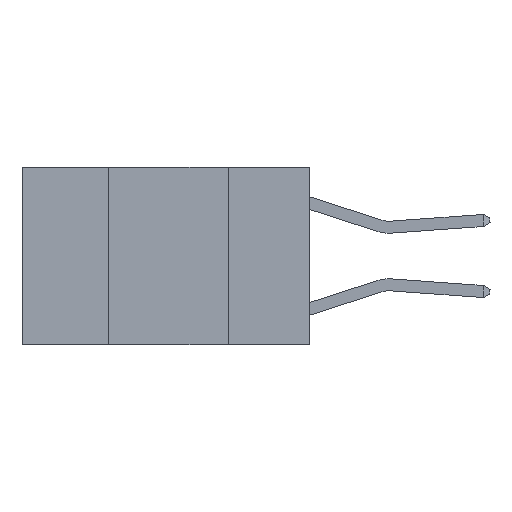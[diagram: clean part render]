
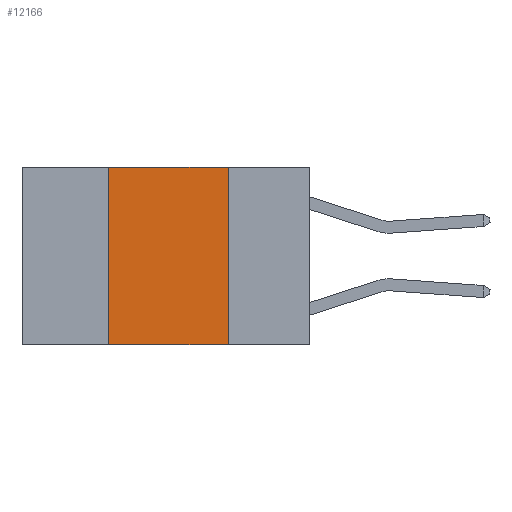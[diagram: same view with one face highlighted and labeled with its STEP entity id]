
A CAD part, left-side view. The second image highlights one B-rep face of the part: STEP entity #12166.
In plain terms, the highlighted planar face has unit normal (-1, 0, 0).
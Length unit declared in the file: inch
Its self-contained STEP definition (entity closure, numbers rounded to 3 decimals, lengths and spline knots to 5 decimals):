
#46 = EDGE_LOOP ( 'NONE', ( #12230, #6119, #9748, #11374 ) ) ;
#489 = EDGE_CURVE ( 'NONE', #6655, #13834, #14466, .T. ) ;
#529 = EDGE_CURVE ( 'NONE', #4726, #6655, #6448, .T. ) ;
#545 = CARTESIAN_POINT ( 'NONE',  ( 0., 0.17, -0.37 ) ) ;
#640 = EDGE_CURVE ( 'NONE', #3314, #13834, #3824, .T. ) ;
#868 = DIRECTION ( 'NONE',  ( 0., 0., -1. ) ) ;
#955 = AXIS2_PLACEMENT_3D ( 'NONE', #13529, #3390, #14388 ) ;
#1019 = CARTESIAN_POINT ( 'NONE',  ( 0., 0.17, 0. ) ) ;
#1156 = PLANE ( 'NONE',  #955 ) ;
#1619 = CARTESIAN_POINT ( 'NONE',  ( 0., 0.17, 0. ) ) ;
#2082 = VECTOR ( 'NONE', #2790, 39.37008 ) ;
#2553 = VECTOR ( 'NONE', #868, 39.37008 ) ;
#2790 = DIRECTION ( 'NONE',  ( 0., -1., 0. ) ) ;
#2953 = CARTESIAN_POINT ( 'NONE',  ( 0., 0.6, 0. ) ) ;
#3314 = VERTEX_POINT ( 'NONE', #9602 ) ;
#3390 = DIRECTION ( 'NONE',  ( 1., 0., 0. ) ) ;
#3824 = LINE ( 'NONE', #13140, #2082 ) ;
#4726 = VERTEX_POINT ( 'NONE', #8680 ) ;
#6119 = ORIENTED_EDGE ( 'NONE', *, *, #529, .F. ) ;
#6448 = LINE ( 'NONE', #2953, #12219 ) ;
#6655 = VERTEX_POINT ( 'NONE', #1619 ) ;
#6734 = LINE ( 'NONE', #14311, #14446 ) ;
#7844 = FACE_OUTER_BOUND ( 'NONE', #46, .T. ) ;
#8495 = EDGE_CURVE ( 'NONE', #3314, #4726, #6734, .T. ) ;
#8680 = CARTESIAN_POINT ( 'NONE',  ( 0., 0.42, 0. ) ) ;
#9602 = CARTESIAN_POINT ( 'NONE',  ( 0., 0.42, -0.37 ) ) ;
#9748 = ORIENTED_EDGE ( 'NONE', *, *, #8495, .F. ) ;
#9950 = DIRECTION ( 'NONE',  ( 0., 0., 1. ) ) ;
#11374 = ORIENTED_EDGE ( 'NONE', *, *, #640, .T. ) ;
#12166 = ADVANCED_FACE ( 'NONE', ( #7844 ), #1156, .F. ) ;
#12219 = VECTOR ( 'NONE', #14033, 39.37008 ) ;
#12230 = ORIENTED_EDGE ( 'NONE', *, *, #489, .F. ) ;
#13140 = CARTESIAN_POINT ( 'NONE',  ( 0., 0.6, -0.37 ) ) ;
#13529 = CARTESIAN_POINT ( 'NONE',  ( 0., 0.6, 0. ) ) ;
#13834 = VERTEX_POINT ( 'NONE', #545 ) ;
#14033 = DIRECTION ( 'NONE',  ( 0., -1., 0. ) ) ;
#14311 = CARTESIAN_POINT ( 'NONE',  ( 0., 0.42, 0. ) ) ;
#14388 = DIRECTION ( 'NONE',  ( 0., 0., -1. ) ) ;
#14446 = VECTOR ( 'NONE', #9950, 39.37008 ) ;
#14466 = LINE ( 'NONE', #1019, #2553 ) ;
